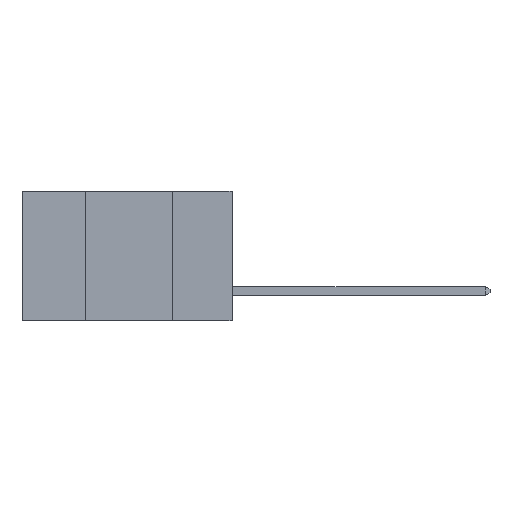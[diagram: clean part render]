
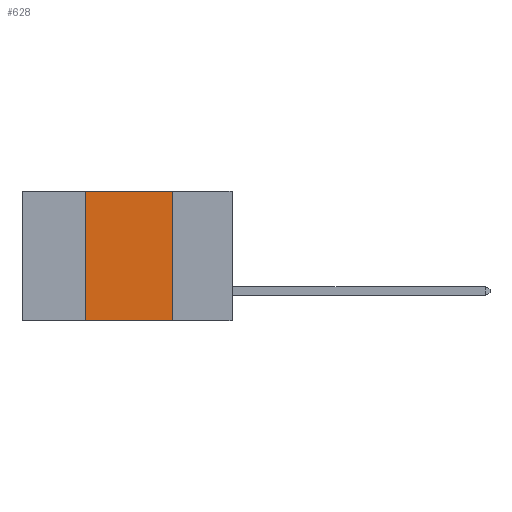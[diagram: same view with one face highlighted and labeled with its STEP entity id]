
A CAD part, left-side view. The second image highlights one B-rep face of the part: STEP entity #628.
In plain terms, the highlighted planar face has unit normal (-1, 0, 0).
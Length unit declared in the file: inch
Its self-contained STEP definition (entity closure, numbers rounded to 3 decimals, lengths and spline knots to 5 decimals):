
#628 = ADVANCED_FACE ( 'NONE', ( #21761 ), #14829, .F. ) ;
#639 = VECTOR ( 'NONE', #25317, 39.37008 ) ;
#2048 = EDGE_CURVE ( 'NONE', #13478, #13242, #15180, .T. ) ;
#2323 = VERTEX_POINT ( 'NONE', #20460 ) ;
#3935 = DIRECTION ( 'NONE',  ( 0., -1., 0. ) ) ;
#4696 = DIRECTION ( 'NONE',  ( 1., 0., 0. ) ) ;
#4960 = DIRECTION ( 'NONE',  ( 0., 0., -1. ) ) ;
#6781 = LINE ( 'NONE', #15401, #639 ) ;
#7450 = ORIENTED_EDGE ( 'NONE', *, *, #22437, .F. ) ;
#8028 = CARTESIAN_POINT ( 'NONE',  ( 0., 0.42, 0. ) ) ;
#8109 = VERTEX_POINT ( 'NONE', #17584 ) ;
#9302 = VECTOR ( 'NONE', #3935, 39.37008 ) ;
#9599 = ORIENTED_EDGE ( 'NONE', *, *, #13988, .F. ) ;
#10421 = AXIS2_PLACEMENT_3D ( 'NONE', #13517, #4696, #4960 ) ;
#13215 = CARTESIAN_POINT ( 'NONE',  ( 0., 0.17, 0. ) ) ;
#13242 = VERTEX_POINT ( 'NONE', #13215 ) ;
#13412 = LINE ( 'NONE', #19032, #18093 ) ;
#13478 = VERTEX_POINT ( 'NONE', #8028 ) ;
#13517 = CARTESIAN_POINT ( 'NONE',  ( 0., 0.6, 0. ) ) ;
#13988 = EDGE_CURVE ( 'NONE', #13242, #8109, #6781, .T. ) ;
#14274 = LINE ( 'NONE', #14500, #19540 ) ;
#14500 = CARTESIAN_POINT ( 'NONE',  ( 0., 0.42, 0. ) ) ;
#14829 = PLANE ( 'NONE',  #10421 ) ;
#15180 = LINE ( 'NONE', #17700, #9302 ) ;
#15401 = CARTESIAN_POINT ( 'NONE',  ( 0., 0.17, 0. ) ) ;
#17584 = CARTESIAN_POINT ( 'NONE',  ( 0., 0.17, -0.37 ) ) ;
#17700 = CARTESIAN_POINT ( 'NONE',  ( 0., 0.6, 0. ) ) ;
#18093 = VECTOR ( 'NONE', #25088, 39.37008 ) ;
#18524 = DIRECTION ( 'NONE',  ( 0., 0., 1. ) ) ;
#19032 = CARTESIAN_POINT ( 'NONE',  ( 0., 0.6, -0.37 ) ) ;
#19540 = VECTOR ( 'NONE', #18524, 39.37008 ) ;
#19828 = ORIENTED_EDGE ( 'NONE', *, *, #2048, .F. ) ;
#20460 = CARTESIAN_POINT ( 'NONE',  ( 0., 0.42, -0.37 ) ) ;
#21761 = FACE_OUTER_BOUND ( 'NONE', #22923, .T. ) ;
#22437 = EDGE_CURVE ( 'NONE', #2323, #13478, #14274, .T. ) ;
#22595 = ORIENTED_EDGE ( 'NONE', *, *, #24446, .T. ) ;
#22923 = EDGE_LOOP ( 'NONE', ( #9599, #19828, #7450, #22595 ) ) ;
#24446 = EDGE_CURVE ( 'NONE', #2323, #8109, #13412, .T. ) ;
#25088 = DIRECTION ( 'NONE',  ( 0., -1., 0. ) ) ;
#25317 = DIRECTION ( 'NONE',  ( 0., 0., -1. ) ) ;
